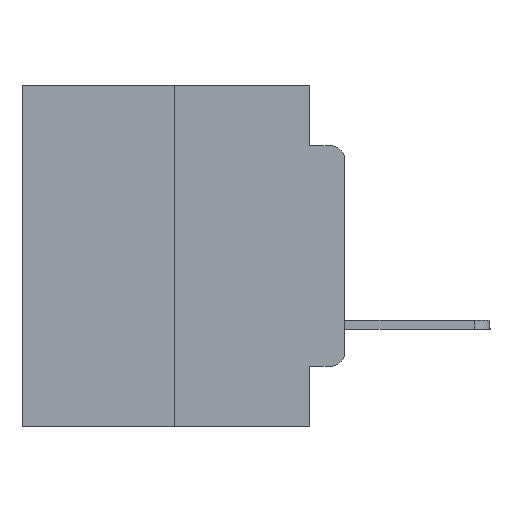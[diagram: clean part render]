
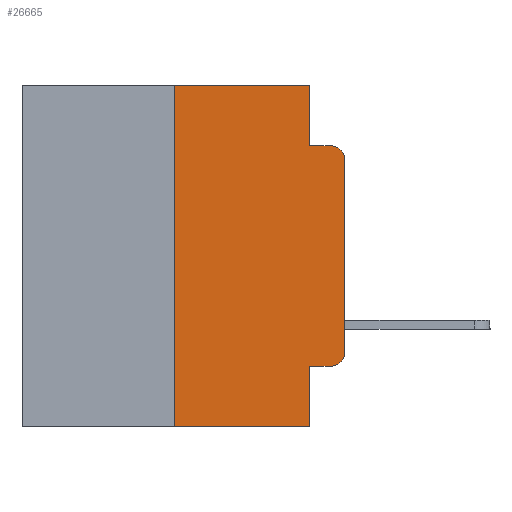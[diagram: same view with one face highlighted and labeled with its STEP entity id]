
A CAD part, left-side view. The second image highlights one B-rep face of the part: STEP entity #26665.
In plain terms, the highlighted planar face has unit normal (-1, 0, 0).
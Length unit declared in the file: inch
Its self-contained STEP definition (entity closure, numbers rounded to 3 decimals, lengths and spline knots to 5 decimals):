
#43 = CARTESIAN_POINT ( 'NONE',  ( 0., 0.25, -0.5 ) ) ;
#175 = ORIENTED_EDGE ( 'NONE', *, *, #6621, .T. ) ;
#509 = ORIENTED_EDGE ( 'NONE', *, *, #13958, .T. ) ;
#639 = EDGE_CURVE ( 'NONE', #9965, #6120, #15202, .T. ) ;
#914 = DIRECTION ( 'NONE',  ( 0., 0., -1. ) ) ;
#1405 = VECTOR ( 'NONE', #13020, 39.37008 ) ;
#1573 = LINE ( 'NONE', #13919, #24259 ) ;
#1633 = LINE ( 'NONE', #25926, #14332 ) ;
#3246 = EDGE_CURVE ( 'NONE', #9742, #15822, #5140, .T. ) ;
#3283 = CARTESIAN_POINT ( 'NONE',  ( 0., 0., 0. ) ) ;
#3339 = EDGE_CURVE ( 'NONE', #5356, #14011, #17635, .T. ) ;
#3583 = CARTESIAN_POINT ( 'NONE',  ( 0., 0.051, -0.5 ) ) ;
#4286 = VECTOR ( 'NONE', #26071, 39.37008 ) ;
#4958 = CARTESIAN_POINT ( 'NONE',  ( 0., 0.02, -0.4115 ) ) ;
#5140 = CIRCLE ( 'NONE', #19040, 0.02 ) ;
#5356 = VERTEX_POINT ( 'NONE', #43 ) ;
#5407 = DIRECTION ( 'NONE',  ( 0., 0., -1. ) ) ;
#5578 = CARTESIAN_POINT ( 'NONE',  ( 0., 0.051, -0.0885 ) ) ;
#5750 = CARTESIAN_POINT ( 'NONE',  ( 0., 0.02, -0.0885 ) ) ;
#5872 = ORIENTED_EDGE ( 'NONE', *, *, #3339, .F. ) ;
#6120 = VERTEX_POINT ( 'NONE', #11788 ) ;
#6372 = DIRECTION ( 'NONE',  ( 0., 0., -1. ) ) ;
#6411 = ORIENTED_EDGE ( 'NONE', *, *, #19955, .F. ) ;
#6449 = EDGE_LOOP ( 'NONE', ( #16057, #24818, #19037, #13267, #15316, #5872, #509, #6411, #175, #21963 ) ) ;
#6621 = EDGE_CURVE ( 'NONE', #26745, #9965, #1573, .T. ) ;
#6797 = FACE_OUTER_BOUND ( 'NONE', #6449, .T. ) ;
#7221 = CARTESIAN_POINT ( 'NONE',  ( 0., 0.051, -0.4115 ) ) ;
#7763 = LINE ( 'NONE', #3283, #24640 ) ;
#8923 = CARTESIAN_POINT ( 'NONE',  ( 0., 0.25, 0. ) ) ;
#9182 = DIRECTION ( 'NONE',  ( 0., -1., 0. ) ) ;
#9497 = CARTESIAN_POINT ( 'NONE',  ( 0., 0.473, 0. ) ) ;
#9504 = CARTESIAN_POINT ( 'NONE',  ( 0., 0., -0.1085 ) ) ;
#9659 = DIRECTION ( 'NONE',  ( 0., -1., 0. ) ) ;
#9742 = VERTEX_POINT ( 'NONE', #9504 ) ;
#9965 = VERTEX_POINT ( 'NONE', #4958 ) ;
#10029 = AXIS2_PLACEMENT_3D ( 'NONE', #23262, #25279, #6372 ) ;
#10767 = CARTESIAN_POINT ( 'NONE',  ( 0., 0.473, 0. ) ) ;
#11236 = VECTOR ( 'NONE', #25887, 39.37008 ) ;
#11788 = CARTESIAN_POINT ( 'NONE',  ( 0., 0., -0.3915 ) ) ;
#13020 = DIRECTION ( 'NONE',  ( 0., 0., -1. ) ) ;
#13141 = DIRECTION ( 'NONE',  ( -1., 0., 0. ) ) ;
#13267 = ORIENTED_EDGE ( 'NONE', *, *, #21452, .F. ) ;
#13444 = CARTESIAN_POINT ( 'NONE',  ( 0., 0.051, 0. ) ) ;
#13919 = CARTESIAN_POINT ( 'NONE',  ( 0., 0.051, -0.4115 ) ) ;
#13958 = EDGE_CURVE ( 'NONE', #5356, #20313, #21689, .T. ) ;
#14011 = VERTEX_POINT ( 'NONE', #25739 ) ;
#14332 = VECTOR ( 'NONE', #5407, 39.37008 ) ;
#14585 = VECTOR ( 'NONE', #9182, 39.37008 ) ;
#14812 = VECTOR ( 'NONE', #9659, 39.37008 ) ;
#15120 = DIRECTION ( 'NONE',  ( 0., 0., -1. ) ) ;
#15166 = CARTESIAN_POINT ( 'NONE',  ( 0., 0.473, -0.5 ) ) ;
#15202 = CIRCLE ( 'NONE', #10029, 0.02 ) ;
#15316 = ORIENTED_EDGE ( 'NONE', *, *, #16788, .F. ) ;
#15482 = VERTEX_POINT ( 'NONE', #13444 ) ;
#15665 = LINE ( 'NONE', #5578, #14812 ) ;
#15822 = VERTEX_POINT ( 'NONE', #5750 ) ;
#16057 = ORIENTED_EDGE ( 'NONE', *, *, #16265, .T. ) ;
#16265 = EDGE_CURVE ( 'NONE', #6120, #9742, #7763, .T. ) ;
#16788 = EDGE_CURVE ( 'NONE', #14011, #15482, #21740, .T. ) ;
#16902 = PLANE ( 'NONE',  #24056 ) ;
#17635 = LINE ( 'NONE', #8923, #11236 ) ;
#17889 = VERTEX_POINT ( 'NONE', #26076 ) ;
#18934 = DIRECTION ( 'NONE',  ( 1., 0., 0. ) ) ;
#19037 = ORIENTED_EDGE ( 'NONE', *, *, #19487, .F. ) ;
#19040 = AXIS2_PLACEMENT_3D ( 'NONE', #23468, #13141, #914 ) ;
#19487 = EDGE_CURVE ( 'NONE', #17889, #15822, #15665, .T. ) ;
#19955 = EDGE_CURVE ( 'NONE', #26745, #20313, #1633, .T. ) ;
#20313 = VERTEX_POINT ( 'NONE', #3583 ) ;
#21452 = EDGE_CURVE ( 'NONE', #15482, #17889, #23478, .T. ) ;
#21689 = LINE ( 'NONE', #15166, #14585 ) ;
#21740 = LINE ( 'NONE', #9497, #4286 ) ;
#21963 = ORIENTED_EDGE ( 'NONE', *, *, #639, .T. ) ;
#22208 = DIRECTION ( 'NONE',  ( 0., -1., 0. ) ) ;
#22318 = DIRECTION ( 'NONE',  ( 0., 0., 1. ) ) ;
#23262 = CARTESIAN_POINT ( 'NONE',  ( 0., 0.02, -0.3915 ) ) ;
#23468 = CARTESIAN_POINT ( 'NONE',  ( 0., 0.02, -0.1085 ) ) ;
#23478 = LINE ( 'NONE', #25364, #1405 ) ;
#24056 = AXIS2_PLACEMENT_3D ( 'NONE', #10767, #18934, #15120 ) ;
#24259 = VECTOR ( 'NONE', #22208, 39.37008 ) ;
#24640 = VECTOR ( 'NONE', #22318, 39.37008 ) ;
#24818 = ORIENTED_EDGE ( 'NONE', *, *, #3246, .T. ) ;
#25279 = DIRECTION ( 'NONE',  ( -1., 0., 0. ) ) ;
#25364 = CARTESIAN_POINT ( 'NONE',  ( 0., 0.051, 0. ) ) ;
#25739 = CARTESIAN_POINT ( 'NONE',  ( 0., 0.25, 0. ) ) ;
#25887 = DIRECTION ( 'NONE',  ( 0., 0., 1. ) ) ;
#25926 = CARTESIAN_POINT ( 'NONE',  ( 0., 0.051, 0. ) ) ;
#26071 = DIRECTION ( 'NONE',  ( 0., -1., 0. ) ) ;
#26076 = CARTESIAN_POINT ( 'NONE',  ( 0., 0.051, -0.0885 ) ) ;
#26665 = ADVANCED_FACE ( 'NONE', ( #6797 ), #16902, .F. ) ;
#26745 = VERTEX_POINT ( 'NONE', #7221 ) ;
